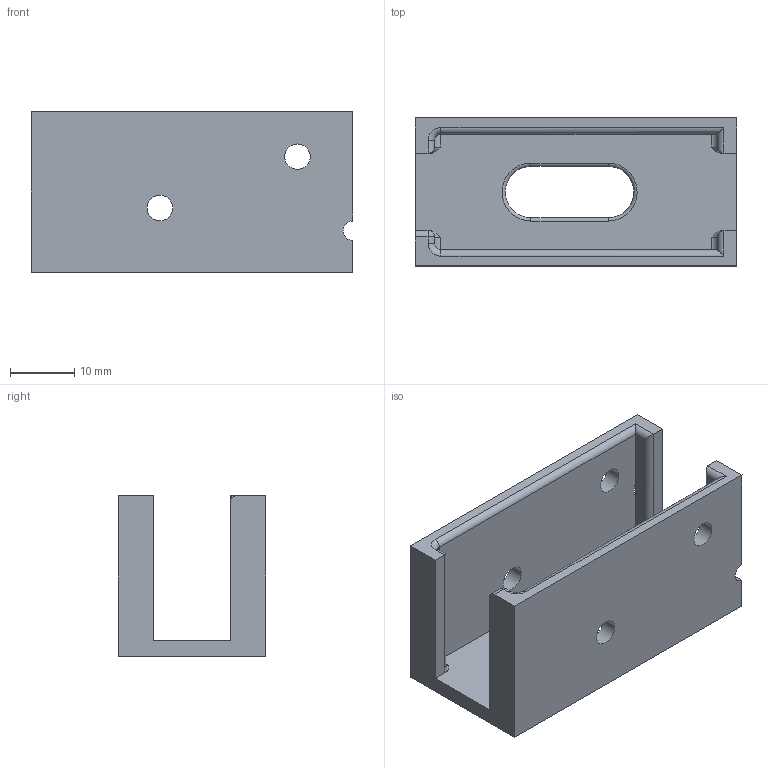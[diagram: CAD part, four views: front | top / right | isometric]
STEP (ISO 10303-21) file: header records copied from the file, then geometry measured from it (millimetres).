
FILE_DESCRIPTION (( 'STEP AP214' ), '1' );
FILE_NAME ('FCG_Module.STEP', '2013-12-17T05:37:26', ( 'elpi' ), ( '' ), 'SwSTEP 2.0', 'SolidWorks 2013', '' );
FILE_SCHEMA (( 'AUTOMOTIVE_DESIGN' ));
Length unit declared in the file: inch
Products named in the file (1): FCG_Module
Bounding box: 50 x 23 x 24.98 mm (x, y, z)
Volume: 8700.5 mm3; surface area: 7667.1 mm2
Topology: 1 solids, 1 shells, 69 faces, 182 edges, 112 vertices
Faces by surface type: cylinder 35, plane 23, torus 10, sphere 1
Entity records: 2199 total; most frequent: CARTESIAN_POINT 412, DIRECTION 378, ORIENTED_EDGE 362, EDGE_CURVE 181, AXIS2_PLACEMENT_3D 138, VERTEX_POINT 112, LINE 102, VECTOR 102
